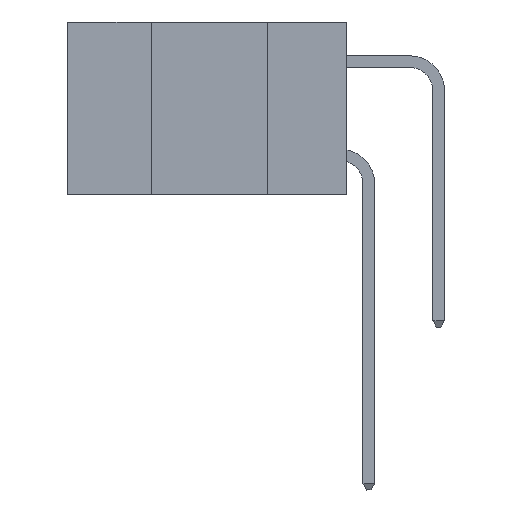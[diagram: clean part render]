
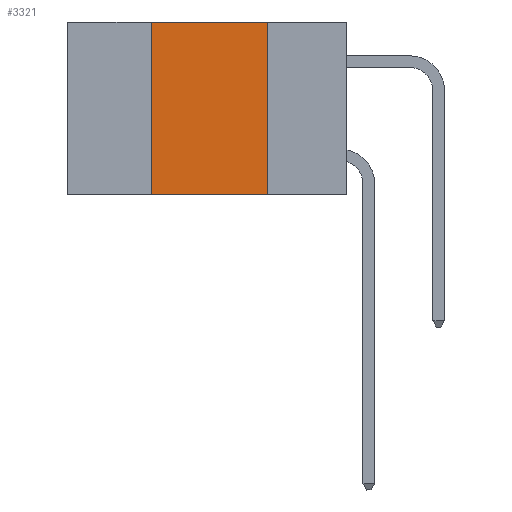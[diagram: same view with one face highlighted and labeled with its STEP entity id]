
A CAD part, left-side view. The second image highlights one B-rep face of the part: STEP entity #3321.
In plain terms, the highlighted planar face has unit normal (-1, 0, 0).
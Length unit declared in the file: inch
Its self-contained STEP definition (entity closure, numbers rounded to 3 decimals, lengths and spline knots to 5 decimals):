
#532 = CARTESIAN_POINT ( 'NONE',  ( 0., 0.17, 0. ) ) ;
#670 = VERTEX_POINT ( 'NONE', #26126 ) ;
#1156 = ORIENTED_EDGE ( 'NONE', *, *, #4169, .F. ) ;
#1278 = PLANE ( 'NONE',  #21797 ) ;
#2112 = CARTESIAN_POINT ( 'NONE',  ( 0., 0.42, 0. ) ) ;
#3321 = ADVANCED_FACE ( 'NONE', ( #21140 ), #1278, .F. ) ;
#3796 = VECTOR ( 'NONE', #9359, 39.37008 ) ;
#4169 = EDGE_CURVE ( 'NONE', #670, #8575, #20396, .T. ) ;
#4319 = CARTESIAN_POINT ( 'NONE',  ( 0., 0.42, -0.37 ) ) ;
#5816 = VECTOR ( 'NONE', #19485, 39.37008 ) ;
#6135 = CARTESIAN_POINT ( 'NONE',  ( 0., 0.17, -0.37 ) ) ;
#7474 = EDGE_CURVE ( 'NONE', #14949, #670, #11915, .T. ) ;
#8322 = DIRECTION ( 'NONE',  ( 0., 0., -1. ) ) ;
#8575 = VERTEX_POINT ( 'NONE', #6135 ) ;
#9359 = DIRECTION ( 'NONE',  ( 0., 0., -1. ) ) ;
#11768 = ORIENTED_EDGE ( 'NONE', *, *, #24649, .T. ) ;
#11915 = LINE ( 'NONE', #22826, #21789 ) ;
#14949 = VERTEX_POINT ( 'NONE', #16996 ) ;
#16273 = LINE ( 'NONE', #2112, #21434 ) ;
#16996 = CARTESIAN_POINT ( 'NONE',  ( 0., 0.42, 0. ) ) ;
#17276 = VERTEX_POINT ( 'NONE', #4319 ) ;
#18289 = DIRECTION ( 'NONE',  ( 0., 0., 1. ) ) ;
#18966 = DIRECTION ( 'NONE',  ( 1., 0., 0. ) ) ;
#19485 = DIRECTION ( 'NONE',  ( 0., -1., 0. ) ) ;
#19741 = EDGE_CURVE ( 'NONE', #17276, #14949, #16273, .T. ) ;
#20396 = LINE ( 'NONE', #532, #3796 ) ;
#21140 = FACE_OUTER_BOUND ( 'NONE', #27400, .T. ) ;
#21434 = VECTOR ( 'NONE', #18289, 39.37008 ) ;
#21651 = LINE ( 'NONE', #26182, #5816 ) ;
#21789 = VECTOR ( 'NONE', #28185, 39.37008 ) ;
#21797 = AXIS2_PLACEMENT_3D ( 'NONE', #27864, #18966, #8322 ) ;
#21998 = ORIENTED_EDGE ( 'NONE', *, *, #19741, .F. ) ;
#22826 = CARTESIAN_POINT ( 'NONE',  ( 0., 0.6, 0. ) ) ;
#24281 = ORIENTED_EDGE ( 'NONE', *, *, #7474, .F. ) ;
#24649 = EDGE_CURVE ( 'NONE', #17276, #8575, #21651, .T. ) ;
#26126 = CARTESIAN_POINT ( 'NONE',  ( 0., 0.17, 0. ) ) ;
#26182 = CARTESIAN_POINT ( 'NONE',  ( 0., 0.6, -0.37 ) ) ;
#27400 = EDGE_LOOP ( 'NONE', ( #1156, #24281, #21998, #11768 ) ) ;
#27864 = CARTESIAN_POINT ( 'NONE',  ( 0., 0.6, 0. ) ) ;
#28185 = DIRECTION ( 'NONE',  ( 0., -1., 0. ) ) ;
